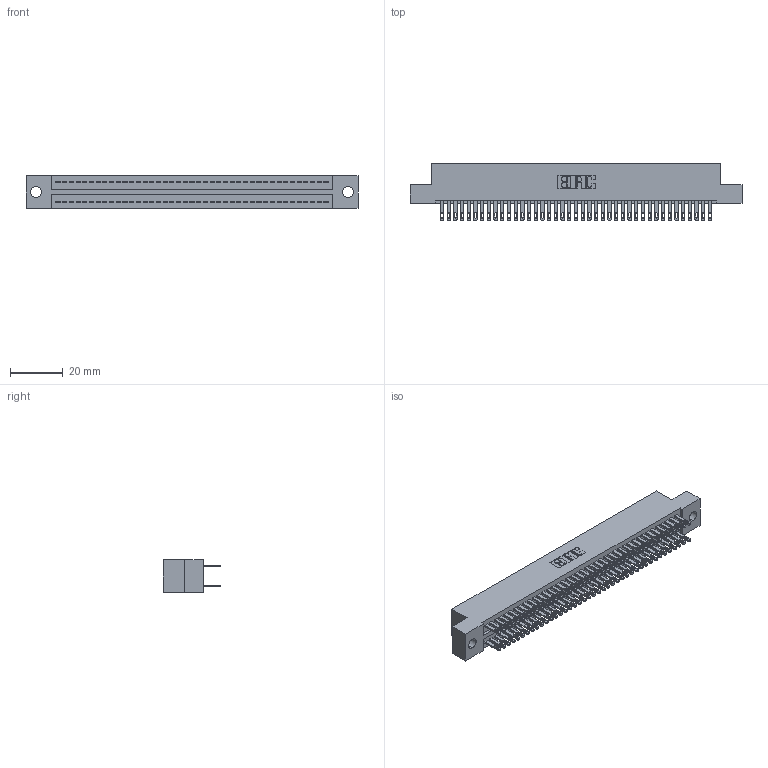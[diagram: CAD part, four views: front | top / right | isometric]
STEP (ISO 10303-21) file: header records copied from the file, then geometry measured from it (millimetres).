
FILE_DESCRIPTION (( 'STEP AP203' ), '1' );
FILE_NAME ('325-082-500-209.STEP', '2020-02-25T04:48:44', ( '' ), ( '' ), 'SwSTEP 2.0', 'SolidWorks 2016', '' );
FILE_SCHEMA (( 'CONFIG_CONTROL_DESIGN' ));
Length unit declared in the file: inch
Products named in the file (3): 325 Part_.160 TH; 325-082-500-209; 325-292-001_325-293-100
Assembly tree (83 placements, depth 2):
  325-082-500-209
    325 Part_.160 TH
    325-292-001_325-293-100  x82
Bounding box: 125.86 x 21.84 x 12.45 mm (x, y, z)
Volume: 16258.4 mm3; surface area: 20432.8 mm2
Topology: 83 solids, 83 shells, 4050 faces, 12365 edges, 8242 vertices
Faces by surface type: plane 2530, cylinder 1520
Entity records: 26439 total; most frequent: CARTESIAN_POINT 4382, ORIENTED_EDGE 4318, DIRECTION 3747, EDGE_CURVE 2159, LINE 2027, VECTOR 2027, VERTEX_POINT 1438, AXIS2_PLACEMENT_3D 860
